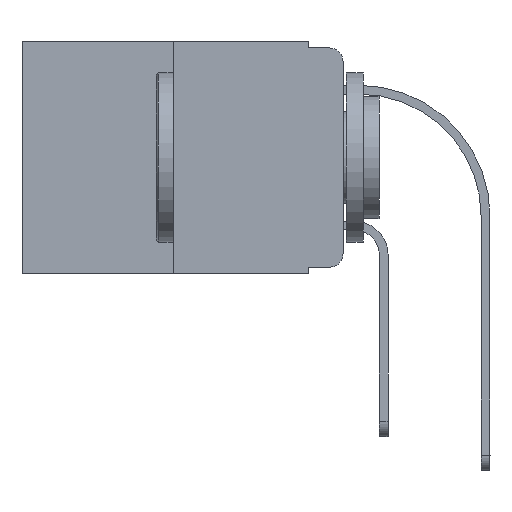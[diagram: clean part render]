
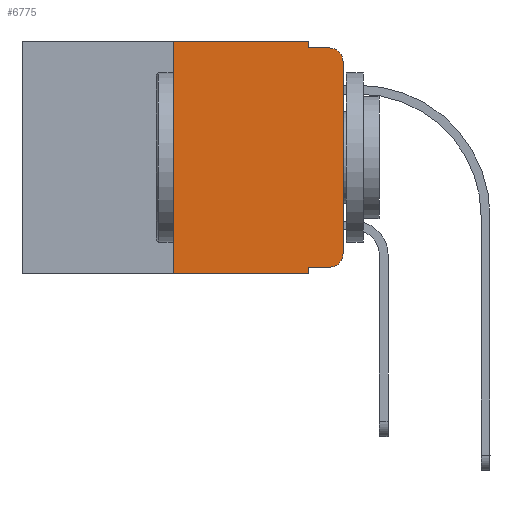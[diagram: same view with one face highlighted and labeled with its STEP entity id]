
A CAD part, left-side view. The second image highlights one B-rep face of the part: STEP entity #6775.
In plain terms, the highlighted planar face has unit normal (-1, 0, 0).
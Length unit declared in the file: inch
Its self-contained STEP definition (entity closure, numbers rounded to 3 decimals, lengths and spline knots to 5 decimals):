
#464 = LINE ( 'NONE', #23570, #5126 ) ;
#627 = CIRCLE ( 'NONE', #24341, 0.02 ) ;
#1398 = AXIS2_PLACEMENT_3D ( 'NONE', #23430, #6369, #21177 ) ;
#2048 = ORIENTED_EDGE ( 'NONE', *, *, #13674, .T. ) ;
#2520 = ORIENTED_EDGE ( 'NONE', *, *, #13487, .F. ) ;
#2952 = VERTEX_POINT ( 'NONE', #8529 ) ;
#3180 = LINE ( 'NONE', #26531, #22545 ) ;
#3198 = VERTEX_POINT ( 'NONE', #20374 ) ;
#3698 = ORIENTED_EDGE ( 'NONE', *, *, #19796, .F. ) ;
#4249 = CARTESIAN_POINT ( 'NONE',  ( 0., 0.051, -0.343 ) ) ;
#4975 = ORIENTED_EDGE ( 'NONE', *, *, #25659, .F. ) ;
#5094 = VERTEX_POINT ( 'NONE', #4249 ) ;
#5126 = VECTOR ( 'NONE', #9014, 39.37008 ) ;
#5883 = CARTESIAN_POINT ( 'NONE',  ( 0., 0.02, -0.01 ) ) ;
#6369 = DIRECTION ( 'NONE',  ( 1., 0., 0. ) ) ;
#6390 = VERTEX_POINT ( 'NONE', #5883 ) ;
#6574 = DIRECTION ( 'NONE',  ( 0., 0., 1. ) ) ;
#6642 = PLANE ( 'NONE',  #1398 ) ;
#6716 = CARTESIAN_POINT ( 'NONE',  ( 0., 0.051, -0.01 ) ) ;
#6775 = ADVANCED_FACE ( 'NONE', ( #25810 ), #6642, .F. ) ;
#7064 = EDGE_CURVE ( 'NONE', #2952, #26159, #14157, .T. ) ;
#7169 = VECTOR ( 'NONE', #14187, 39.37008 ) ;
#7550 = CARTESIAN_POINT ( 'NONE',  ( 0., 0., -0.03 ) ) ;
#7731 = VERTEX_POINT ( 'NONE', #25195 ) ;
#7845 = DIRECTION ( 'NONE',  ( 0., 0., -1. ) ) ;
#7870 = VERTEX_POINT ( 'NONE', #6716 ) ;
#8180 = CARTESIAN_POINT ( 'NONE',  ( 0., 0.051, -0.333 ) ) ;
#8529 = CARTESIAN_POINT ( 'NONE',  ( 0., 0.25, -0.343 ) ) ;
#8742 = VERTEX_POINT ( 'NONE', #15690 ) ;
#9014 = DIRECTION ( 'NONE',  ( 0., -1., 0. ) ) ;
#9536 = CARTESIAN_POINT ( 'NONE',  ( 0., 0.051, 0. ) ) ;
#9959 = CARTESIAN_POINT ( 'NONE',  ( 0., 0.02, -0.03 ) ) ;
#9979 = DIRECTION ( 'NONE',  ( 0., 0., -1. ) ) ;
#10245 = DIRECTION ( 'NONE',  ( 0., 0., -1. ) ) ;
#10263 = CARTESIAN_POINT ( 'NONE',  ( 0., 0.02, -0.313 ) ) ;
#10437 = CIRCLE ( 'NONE', #24737, 0.02 ) ;
#11065 = CARTESIAN_POINT ( 'NONE',  ( 0., 0.25, 0. ) ) ;
#11312 = LINE ( 'NONE', #15515, #17712 ) ;
#12471 = LINE ( 'NONE', #21259, #15430 ) ;
#12909 = EDGE_CURVE ( 'NONE', #2952, #5094, #464, .T. ) ;
#13487 = EDGE_CURVE ( 'NONE', #8742, #7870, #26861, .T. ) ;
#13674 = EDGE_CURVE ( 'NONE', #18080, #6390, #10437, .T. ) ;
#13921 = VECTOR ( 'NONE', #22717, 39.37008 ) ;
#14157 = LINE ( 'NONE', #18798, #13921 ) ;
#14163 = ORIENTED_EDGE ( 'NONE', *, *, #12909, .T. ) ;
#14187 = DIRECTION ( 'NONE',  ( 0., -1., 0. ) ) ;
#15430 = VECTOR ( 'NONE', #10245, 39.37008 ) ;
#15515 = CARTESIAN_POINT ( 'NONE',  ( 0., 0., 0. ) ) ;
#15690 = CARTESIAN_POINT ( 'NONE',  ( 0., 0.051, 0. ) ) ;
#15903 = DIRECTION ( 'NONE',  ( 0., -1., 0. ) ) ;
#15952 = DIRECTION ( 'NONE',  ( 0., 0., -1. ) ) ;
#16023 = ORIENTED_EDGE ( 'NONE', *, *, #22940, .F. ) ;
#16218 = ORIENTED_EDGE ( 'NONE', *, *, #23111, .T. ) ;
#16401 = DIRECTION ( 'NONE',  ( -1., 0., 0. ) ) ;
#16408 = VECTOR ( 'NONE', #25391, 39.37008 ) ;
#16840 = CARTESIAN_POINT ( 'NONE',  ( 0., 0.473, 0. ) ) ;
#17712 = VECTOR ( 'NONE', #6574, 39.37008 ) ;
#18080 = VERTEX_POINT ( 'NONE', #7550 ) ;
#18798 = CARTESIAN_POINT ( 'NONE',  ( 0., 0.25, 0. ) ) ;
#19363 = CARTESIAN_POINT ( 'NONE',  ( 0., 0.051, -0.333 ) ) ;
#19796 = EDGE_CURVE ( 'NONE', #7870, #6390, #3180, .T. ) ;
#20374 = CARTESIAN_POINT ( 'NONE',  ( 0., 0.02, -0.333 ) ) ;
#20476 = ORIENTED_EDGE ( 'NONE', *, *, #7064, .F. ) ;
#21135 = VECTOR ( 'NONE', #15952, 39.37008 ) ;
#21177 = DIRECTION ( 'NONE',  ( 0., 0., -1. ) ) ;
#21259 = CARTESIAN_POINT ( 'NONE',  ( 0., 0.051, 0. ) ) ;
#21805 = EDGE_CURVE ( 'NONE', #21945, #3198, #24840, .T. ) ;
#21945 = VERTEX_POINT ( 'NONE', #19363 ) ;
#22115 = ORIENTED_EDGE ( 'NONE', *, *, #22199, .T. ) ;
#22163 = ORIENTED_EDGE ( 'NONE', *, *, #21805, .T. ) ;
#22199 = EDGE_CURVE ( 'NONE', #3198, #7731, #627, .T. ) ;
#22545 = VECTOR ( 'NONE', #15903, 39.37008 ) ;
#22717 = DIRECTION ( 'NONE',  ( 0., 0., 1. ) ) ;
#22940 = EDGE_CURVE ( 'NONE', #21945, #5094, #12471, .T. ) ;
#23111 = EDGE_CURVE ( 'NONE', #7731, #18080, #11312, .T. ) ;
#23430 = CARTESIAN_POINT ( 'NONE',  ( 0., 0.473, 0. ) ) ;
#23570 = CARTESIAN_POINT ( 'NONE',  ( 0., 0.473, -0.343 ) ) ;
#24239 = EDGE_LOOP ( 'NONE', ( #16218, #2048, #3698, #2520, #4975, #20476, #14163, #16023, #22163, #22115 ) ) ;
#24341 = AXIS2_PLACEMENT_3D ( 'NONE', #10263, #16401, #9979 ) ;
#24737 = AXIS2_PLACEMENT_3D ( 'NONE', #9959, #26985, #7845 ) ;
#24840 = LINE ( 'NONE', #8180, #7169 ) ;
#25195 = CARTESIAN_POINT ( 'NONE',  ( 0., 0., -0.313 ) ) ;
#25391 = DIRECTION ( 'NONE',  ( 0., -1., 0. ) ) ;
#25659 = EDGE_CURVE ( 'NONE', #26159, #8742, #27440, .T. ) ;
#25810 = FACE_OUTER_BOUND ( 'NONE', #24239, .T. ) ;
#26159 = VERTEX_POINT ( 'NONE', #11065 ) ;
#26531 = CARTESIAN_POINT ( 'NONE',  ( 0., 0.051, -0.01 ) ) ;
#26861 = LINE ( 'NONE', #9536, #21135 ) ;
#26985 = DIRECTION ( 'NONE',  ( -1., 0., 0. ) ) ;
#27440 = LINE ( 'NONE', #16840, #16408 ) ;
